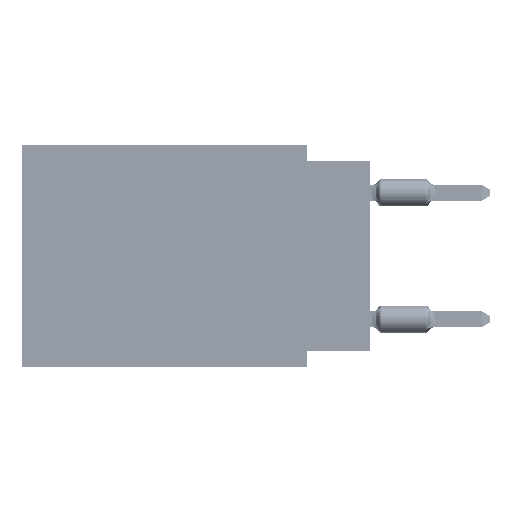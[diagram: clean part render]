
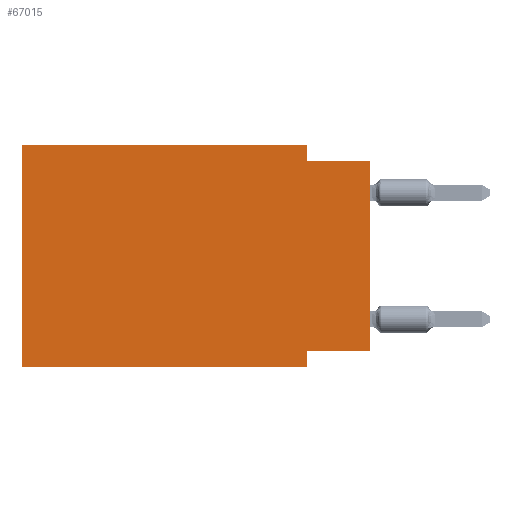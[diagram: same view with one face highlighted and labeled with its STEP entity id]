
A CAD part, left-side view. The second image highlights one B-rep face of the part: STEP entity #67015.
In plain terms, the highlighted planar face has unit normal (-1, 0, 0).
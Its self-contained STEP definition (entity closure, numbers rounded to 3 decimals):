
#99 = ORIENTED_EDGE ( 'NONE', *, *, #2891, .F. ) ;
#312 = CARTESIAN_POINT ( 'NONE',  ( 0., 2.54, 0. ) ) ;
#1446 = VERTEX_POINT ( 'NONE', #51699 ) ;
#2300 = VERTEX_POINT ( 'NONE', #51080 ) ;
#2354 = DIRECTION ( 'NONE',  ( 0., 0., -1. ) ) ;
#2891 = EDGE_CURVE ( 'NONE', #2300, #23877, #61167, .T. ) ;
#5015 = CARTESIAN_POINT ( 'NONE',  ( 0., 13.97, 0. ) ) ;
#5253 = DIRECTION ( 'NONE',  ( 0., 0., 1. ) ) ;
#5976 = CARTESIAN_POINT ( 'NONE',  ( 0., 0., 0. ) ) ;
#7082 = DIRECTION ( 'NONE',  ( 0., 0., 1. ) ) ;
#9598 = DIRECTION ( 'NONE',  ( 0., 0., -1. ) ) ;
#10752 = CARTESIAN_POINT ( 'NONE',  ( 0., 0., -0.635 ) ) ;
#13224 = EDGE_LOOP ( 'NONE', ( #33903, #60384, #63978, #71409, #99, #25463, #26010, #26738 ) ) ;
#15456 = VECTOR ( 'NONE', #23082, 1000. ) ;
#16165 = VERTEX_POINT ( 'NONE', #312 ) ;
#16683 = VECTOR ( 'NONE', #5253, 1000. ) ;
#18296 = CARTESIAN_POINT ( 'NONE',  ( 0., 0., -8.255 ) ) ;
#19402 = EDGE_CURVE ( 'NONE', #1446, #70728, #45592, .T. ) ;
#19566 = VECTOR ( 'NONE', #59958, 1000. ) ;
#19587 = LINE ( 'NONE', #41957, #65754 ) ;
#20243 = CARTESIAN_POINT ( 'NONE',  ( 0., 13.97, 0. ) ) ;
#21758 = LINE ( 'NONE', #10752, #19566 ) ;
#22929 = VERTEX_POINT ( 'NONE', #47109 ) ;
#23082 = DIRECTION ( 'NONE',  ( 0., 1., 0. ) ) ;
#23432 = DIRECTION ( 'NONE',  ( 0., 0., -1. ) ) ;
#23877 = VERTEX_POINT ( 'NONE', #43601 ) ;
#24436 = CARTESIAN_POINT ( 'NONE',  ( 0., 2.54, -8.89 ) ) ;
#25093 = LINE ( 'NONE', #58139, #60093 ) ;
#25463 = ORIENTED_EDGE ( 'NONE', *, *, #27937, .T. ) ;
#25748 = FACE_OUTER_BOUND ( 'NONE', #13224, .T. ) ;
#26010 = ORIENTED_EDGE ( 'NONE', *, *, #58440, .F. ) ;
#26738 = ORIENTED_EDGE ( 'NONE', *, *, #55607, .F. ) ;
#27937 = EDGE_CURVE ( 'NONE', #2300, #56094, #39026, .T. ) ;
#31249 = CARTESIAN_POINT ( 'NONE',  ( 0., 0., -0.635 ) ) ;
#31958 = DIRECTION ( 'NONE',  ( 0., -1., 0. ) ) ;
#33879 = CARTESIAN_POINT ( 'NONE',  ( 0., 13.97, -8.89 ) ) ;
#33903 = ORIENTED_EDGE ( 'NONE', *, *, #19402, .T. ) ;
#34741 = VECTOR ( 'NONE', #7082, 1000. ) ;
#37472 = DIRECTION ( 'NONE',  ( 1., 0., 0. ) ) ;
#39026 = LINE ( 'NONE', #33879, #40501 ) ;
#39381 = DIRECTION ( 'NONE',  ( 0., -1., 0. ) ) ;
#40501 = VECTOR ( 'NONE', #39381, 1000. ) ;
#41957 = CARTESIAN_POINT ( 'NONE',  ( 0., 13.97, 0. ) ) ;
#43099 = VERTEX_POINT ( 'NONE', #56161 ) ;
#43601 = CARTESIAN_POINT ( 'NONE',  ( 0., 13.97, 0. ) ) ;
#45592 = LINE ( 'NONE', #5976, #16683 ) ;
#47109 = CARTESIAN_POINT ( 'NONE',  ( 0., 2.54, -8.255 ) ) ;
#50972 = LINE ( 'NONE', #56492, #59908 ) ;
#51080 = CARTESIAN_POINT ( 'NONE',  ( 0., 13.97, -8.89 ) ) ;
#51699 = CARTESIAN_POINT ( 'NONE',  ( 0., 0., -8.255 ) ) ;
#51961 = EDGE_CURVE ( 'NONE', #16165, #43099, #50972, .T. ) ;
#52568 = AXIS2_PLACEMENT_3D ( 'NONE', #20243, #37472, #9598 ) ;
#53650 = PLANE ( 'NONE',  #52568 ) ;
#55607 = EDGE_CURVE ( 'NONE', #1446, #22929, #68584, .T. ) ;
#56094 = VERTEX_POINT ( 'NONE', #24436 ) ;
#56161 = CARTESIAN_POINT ( 'NONE',  ( 0., 2.54, -0.635 ) ) ;
#56492 = CARTESIAN_POINT ( 'NONE',  ( 0., 2.54, 0. ) ) ;
#56607 = EDGE_CURVE ( 'NONE', #23877, #16165, #19587, .T. ) ;
#58139 = CARTESIAN_POINT ( 'NONE',  ( 0., 2.54, -8.89 ) ) ;
#58440 = EDGE_CURVE ( 'NONE', #22929, #56094, #25093, .T. ) ;
#59908 = VECTOR ( 'NONE', #23432, 1000. ) ;
#59958 = DIRECTION ( 'NONE',  ( 0., -1., 0. ) ) ;
#60093 = VECTOR ( 'NONE', #2354, 1000. ) ;
#60384 = ORIENTED_EDGE ( 'NONE', *, *, #64832, .F. ) ;
#61167 = LINE ( 'NONE', #5015, #34741 ) ;
#63978 = ORIENTED_EDGE ( 'NONE', *, *, #51961, .F. ) ;
#64832 = EDGE_CURVE ( 'NONE', #43099, #70728, #21758, .T. ) ;
#65754 = VECTOR ( 'NONE', #31958, 1000. ) ;
#67015 = ADVANCED_FACE ( 'NONE', ( #25748 ), #53650, .F. ) ;
#68584 = LINE ( 'NONE', #18296, #15456 ) ;
#70728 = VERTEX_POINT ( 'NONE', #31249 ) ;
#71409 = ORIENTED_EDGE ( 'NONE', *, *, #56607, .F. ) ;
